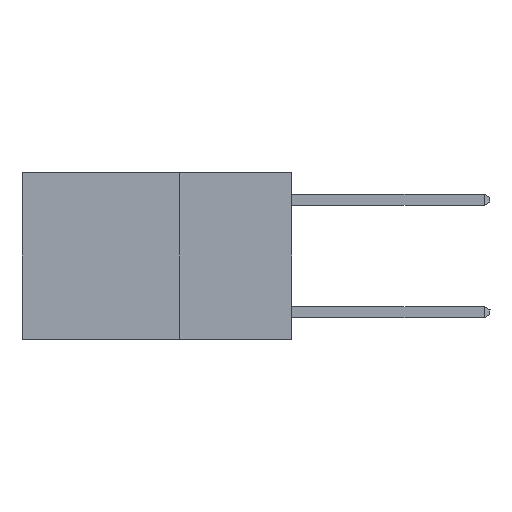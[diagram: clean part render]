
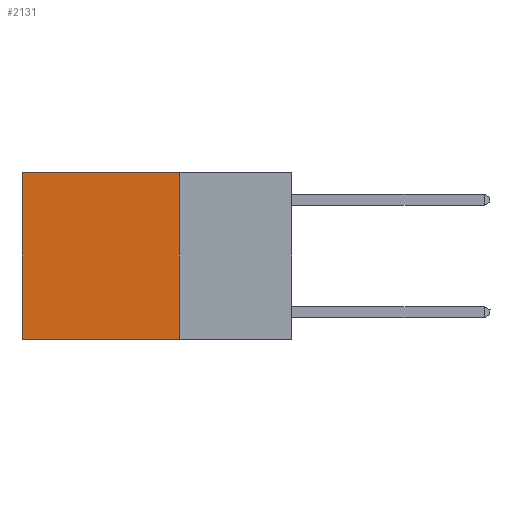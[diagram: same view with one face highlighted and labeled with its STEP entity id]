
A CAD part, left-side view. The second image highlights one B-rep face of the part: STEP entity #2131.
In plain terms, the highlighted planar face has unit normal (-1, 0, 0).
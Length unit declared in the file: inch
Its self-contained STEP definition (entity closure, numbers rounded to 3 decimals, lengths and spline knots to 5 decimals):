
#379 = VECTOR ( 'NONE', #10471, 39.37008 ) ;
#982 = ORIENTED_EDGE ( 'NONE', *, *, #7667, .T. ) ;
#993 = LINE ( 'NONE', #11061, #7742 ) ;
#1002 = VECTOR ( 'NONE', #2764, 39.37008 ) ;
#1535 = ORIENTED_EDGE ( 'NONE', *, *, #4618, .F. ) ;
#1753 = CARTESIAN_POINT ( 'NONE',  ( 0.2625, 0.6, 0. ) ) ;
#1867 = CARTESIAN_POINT ( 'NONE',  ( 0.2625, 0.25, 0. ) ) ;
#1956 = VERTEX_POINT ( 'NONE', #2282 ) ;
#2131 = ADVANCED_FACE ( 'NONE', ( #4616 ), #10313, .F. ) ;
#2282 = CARTESIAN_POINT ( 'NONE',  ( 0.2625, 0.25, 0. ) ) ;
#2510 = CARTESIAN_POINT ( 'NONE',  ( 0.2625, 0.25, 0. ) ) ;
#2543 = CARTESIAN_POINT ( 'NONE',  ( 0.2625, 0.25, -0.37 ) ) ;
#2764 = DIRECTION ( 'NONE',  ( 0., 1., 0. ) ) ;
#2928 = VECTOR ( 'NONE', #3401, 39.37008 ) ;
#3387 = EDGE_CURVE ( 'NONE', #1956, #9418, #993, .T. ) ;
#3401 = DIRECTION ( 'NONE',  ( 0., 1., 0. ) ) ;
#4421 = CARTESIAN_POINT ( 'NONE',  ( 0.2625, 0.6, 0. ) ) ;
#4440 = ORIENTED_EDGE ( 'NONE', *, *, #6597, .T. ) ;
#4616 = FACE_OUTER_BOUND ( 'NONE', #7638, .T. ) ;
#4618 = EDGE_CURVE ( 'NONE', #9418, #4671, #7580, .T. ) ;
#4671 = VERTEX_POINT ( 'NONE', #7836 ) ;
#5127 = LINE ( 'NONE', #4421, #379 ) ;
#5140 = DIRECTION ( 'NONE',  ( 1., 0., 0. ) ) ;
#5822 = CARTESIAN_POINT ( 'NONE',  ( 0.2625, 0.25, -0.37 ) ) ;
#5991 = LINE ( 'NONE', #1867, #1002 ) ;
#6597 = EDGE_CURVE ( 'NONE', #1956, #11025, #5991, .T. ) ;
#7580 = LINE ( 'NONE', #2543, #2928 ) ;
#7638 = EDGE_LOOP ( 'NONE', ( #982, #1535, #11064, #4440 ) ) ;
#7667 = EDGE_CURVE ( 'NONE', #11025, #4671, #5127, .T. ) ;
#7742 = VECTOR ( 'NONE', #10250, 39.37008 ) ;
#7836 = CARTESIAN_POINT ( 'NONE',  ( 0.2625, 0.6, -0.37 ) ) ;
#9418 = VERTEX_POINT ( 'NONE', #5822 ) ;
#10250 = DIRECTION ( 'NONE',  ( 0., 0., -1. ) ) ;
#10313 = PLANE ( 'NONE',  #10335 ) ;
#10335 = AXIS2_PLACEMENT_3D ( 'NONE', #2510, #5140, #11161 ) ;
#10471 = DIRECTION ( 'NONE',  ( 0., 0., -1. ) ) ;
#11025 = VERTEX_POINT ( 'NONE', #1753 ) ;
#11061 = CARTESIAN_POINT ( 'NONE',  ( 0.2625, 0.25, 0. ) ) ;
#11064 = ORIENTED_EDGE ( 'NONE', *, *, #3387, .F. ) ;
#11161 = DIRECTION ( 'NONE',  ( 0., 0., -1. ) ) ;
